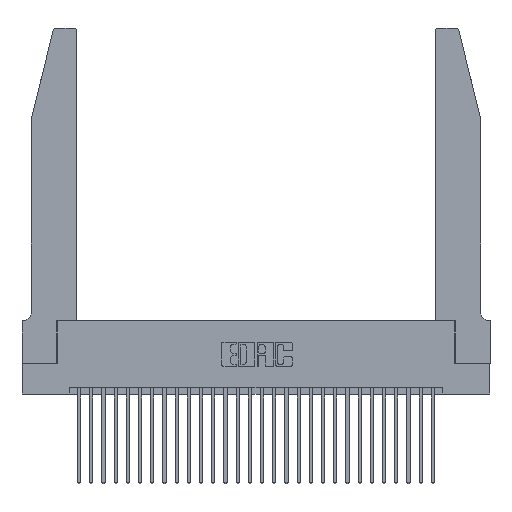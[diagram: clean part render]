
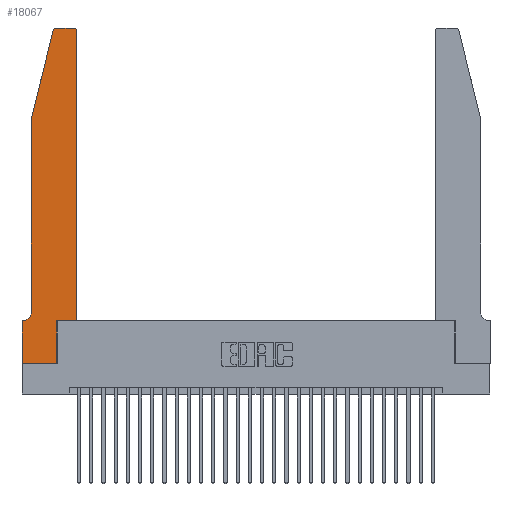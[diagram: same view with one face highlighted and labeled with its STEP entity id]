
A CAD part, top view. The second image highlights one B-rep face of the part: STEP entity #18067.
In plain terms, the highlighted planar face has unit normal (0, 0, 1).
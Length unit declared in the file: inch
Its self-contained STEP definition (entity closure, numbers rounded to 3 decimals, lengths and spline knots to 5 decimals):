
#1061 = VECTOR ( 'NONE', #6796, 39.37008 ) ;
#1632 = ORIENTED_EDGE ( 'NONE', *, *, #29588, .T. ) ;
#1982 = LINE ( 'NONE', #19739, #25883 ) ;
#2063 = CARTESIAN_POINT ( 'NONE',  ( 0.2605, 2.75, 0.37 ) ) ;
#2290 = ORIENTED_EDGE ( 'NONE', *, *, #21706, .T. ) ;
#3856 = CARTESIAN_POINT ( 'NONE',  ( 0.4205, 2.72, 0.37 ) ) ;
#4141 = DIRECTION ( 'NONE',  ( 0., -1., 0. ) ) ;
#5134 = VECTOR ( 'NONE', #19343, 39.37008 ) ;
#5338 = DIRECTION ( 'NONE',  ( 1., 0., 0. ) ) ;
#5572 = DIRECTION ( 'NONE',  ( -0.239, -0.971, 0. ) ) ;
#6156 = CARTESIAN_POINT ( 'NONE',  ( 0.4205, 2.75, 0.37 ) ) ;
#6493 = EDGE_CURVE ( 'NONE', #22655, #26320, #8952, .T. ) ;
#6659 = ORIENTED_EDGE ( 'NONE', *, *, #19389, .T. ) ;
#6733 = CARTESIAN_POINT ( 'NONE',  ( 0.284, 2.72, 0.37 ) ) ;
#6796 = DIRECTION ( 'NONE',  ( 0., 1., 0. ) ) ;
#7118 = AXIS2_PLACEMENT_3D ( 'NONE', #3856, #22224, #20282 ) ;
#7209 = LINE ( 'NONE', #25021, #1061 ) ;
#7869 = VERTEX_POINT ( 'NONE', #20244 ) ;
#8252 = CARTESIAN_POINT ( 'NONE',  ( 0.4505, 0.35, 0.37 ) ) ;
#8328 = AXIS2_PLACEMENT_3D ( 'NONE', #6733, #25265, #27579 ) ;
#8332 = DIRECTION ( 'NONE',  ( -1., 0., 0. ) ) ;
#8952 = LINE ( 'NONE', #11837, #28166 ) ;
#9017 = VERTEX_POINT ( 'NONE', #27501 ) ;
#9073 = VERTEX_POINT ( 'NONE', #13905 ) ;
#9078 = ORIENTED_EDGE ( 'NONE', *, *, #29546, .T. ) ;
#9203 = VECTOR ( 'NONE', #5338, 39.37008 ) ;
#9362 = VECTOR ( 'NONE', #11116, 39.37008 ) ;
#9477 = LINE ( 'NONE', #23958, #5134 ) ;
#9739 = EDGE_CURVE ( 'NONE', #13799, #22655, #9477, .T. ) ;
#9855 = CARTESIAN_POINT ( 'NONE',  ( 0., 0., 0.37 ) ) ;
#10223 = CARTESIAN_POINT ( 'NONE',  ( 0.25487, 2.72718, 0.37 ) ) ;
#10576 = ORIENTED_EDGE ( 'NONE', *, *, #16892, .T. ) ;
#11116 = DIRECTION ( 'NONE',  ( -1., 0., 0. ) ) ;
#11837 = CARTESIAN_POINT ( 'NONE',  ( 0.4505, 0.35, 0.37 ) ) ;
#12440 = CARTESIAN_POINT ( 'NONE',  ( 0.0755, 2., 0.37 ) ) ;
#12889 = CARTESIAN_POINT ( 'NONE',  ( 0.0055, 0.42, 0.37 ) ) ;
#13212 = VECTOR ( 'NONE', #4141, 39.37008 ) ;
#13799 = VERTEX_POINT ( 'NONE', #24764 ) ;
#13905 = CARTESIAN_POINT ( 'NONE',  ( 0., 0.35, 0.37 ) ) ;
#14113 = CIRCLE ( 'NONE', #8328, 0.03 ) ;
#14149 = EDGE_CURVE ( 'NONE', #21076, #9017, #16489, .T. ) ;
#14262 = CARTESIAN_POINT ( 'NONE',  ( 0.4505, 2.72, 0.37 ) ) ;
#14494 = VERTEX_POINT ( 'NONE', #6156 ) ;
#14792 = VECTOR ( 'NONE', #5572, 39.37008 ) ;
#15273 = ORIENTED_EDGE ( 'NONE', *, *, #6493, .T. ) ;
#15652 = CARTESIAN_POINT ( 'NONE',  ( 0., 0., 0.37 ) ) ;
#15943 = DIRECTION ( 'NONE',  ( 0., 0., 1. ) ) ;
#16089 = CIRCLE ( 'NONE', #7118, 0.03 ) ;
#16137 = ORIENTED_EDGE ( 'NONE', *, *, #25163, .T. ) ;
#16489 = CIRCLE ( 'NONE', #19311, 0.07 ) ;
#16553 = VERTEX_POINT ( 'NONE', #10223 ) ;
#16892 = EDGE_CURVE ( 'NONE', #16553, #23480, #28209, .T. ) ;
#17016 = ORIENTED_EDGE ( 'NONE', *, *, #29113, .T. ) ;
#17383 = DIRECTION ( 'NONE',  ( 0., 0., -1. ) ) ;
#17653 = PLANE ( 'NONE',  #24280 ) ;
#17777 = CARTESIAN_POINT ( 'NONE',  ( 0.0755, 0.42, 0.37 ) ) ;
#17938 = CARTESIAN_POINT ( 'NONE',  ( 0.0755, 2., 0.37 ) ) ;
#18067 = ADVANCED_FACE ( 'NONE', ( #21956 ), #17653, .T. ) ;
#19130 = CARTESIAN_POINT ( 'NONE',  ( 0.0755, 2., 0.37 ) ) ;
#19247 = ORIENTED_EDGE ( 'NONE', *, *, #14149, .T. ) ;
#19311 = AXIS2_PLACEMENT_3D ( 'NONE', #12889, #17383, #24340 ) ;
#19343 = DIRECTION ( 'NONE',  ( 1., 0., 0. ) ) ;
#19389 = EDGE_CURVE ( 'NONE', #23480, #21076, #27340, .T. ) ;
#19671 = DIRECTION ( 'NONE',  ( 0., 1., 0. ) ) ;
#19739 = CARTESIAN_POINT ( 'NONE',  ( 0.0755, 0.35, 0.37 ) ) ;
#20244 = CARTESIAN_POINT ( 'NONE',  ( 0., 0., 0.37 ) ) ;
#20282 = DIRECTION ( 'NONE',  ( 1., 0., 0. ) ) ;
#20505 = DIRECTION ( 'NONE',  ( 1., 0., 0. ) ) ;
#20700 = VECTOR ( 'NONE', #23064, 39.37008 ) ;
#21076 = VERTEX_POINT ( 'NONE', #17777 ) ;
#21661 = ORIENTED_EDGE ( 'NONE', *, *, #25024, .T. ) ;
#21706 = EDGE_CURVE ( 'NONE', #9073, #7869, #26887, .T. ) ;
#21956 = FACE_OUTER_BOUND ( 'NONE', #27781, .T. ) ;
#22224 = DIRECTION ( 'NONE',  ( 0., 0., 1. ) ) ;
#22655 = VERTEX_POINT ( 'NONE', #8252 ) ;
#23064 = DIRECTION ( 'NONE',  ( 0., -1., 0. ) ) ;
#23480 = VERTEX_POINT ( 'NONE', #19130 ) ;
#23958 = CARTESIAN_POINT ( 'NONE',  ( 0.4505, 0.35, 0.37 ) ) ;
#24066 = LINE ( 'NONE', #9855, #9203 ) ;
#24280 = AXIS2_PLACEMENT_3D ( 'NONE', #27836, #15943, #20505 ) ;
#24340 = DIRECTION ( 'NONE',  ( -1., 0., 0. ) ) ;
#24466 = EDGE_CURVE ( 'NONE', #26320, #14494, #16089, .T. ) ;
#24531 = VERTEX_POINT ( 'NONE', #24996 ) ;
#24764 = CARTESIAN_POINT ( 'NONE',  ( 0.2865, 0.35, 0.37 ) ) ;
#24996 = CARTESIAN_POINT ( 'NONE',  ( 0.2865, 0., 0.37 ) ) ;
#25021 = CARTESIAN_POINT ( 'NONE',  ( 0.2865, 0.35, 0.37 ) ) ;
#25024 = EDGE_CURVE ( 'NONE', #7869, #24531, #24066, .T. ) ;
#25163 = EDGE_CURVE ( 'NONE', #9017, #9073, #1982, .T. ) ;
#25265 = DIRECTION ( 'NONE',  ( 0., 0., 1. ) ) ;
#25883 = VECTOR ( 'NONE', #8332, 39.37008 ) ;
#26320 = VERTEX_POINT ( 'NONE', #14262 ) ;
#26405 = LINE ( 'NONE', #2063, #9362 ) ;
#26887 = LINE ( 'NONE', #15652, #20700 ) ;
#26948 = CARTESIAN_POINT ( 'NONE',  ( 0.284, 2.75, 0.37 ) ) ;
#27340 = LINE ( 'NONE', #17938, #13212 ) ;
#27501 = CARTESIAN_POINT ( 'NONE',  ( 0.0055, 0.35, 0.37 ) ) ;
#27579 = DIRECTION ( 'NONE',  ( 1., 0., 0. ) ) ;
#27781 = EDGE_LOOP ( 'NONE', ( #9078, #17016, #10576, #6659, #19247, #16137, #2290, #21661, #1632, #29381, #15273, #29273 ) ) ;
#27836 = CARTESIAN_POINT ( 'NONE',  ( 0., 0.35, 0.37 ) ) ;
#28166 = VECTOR ( 'NONE', #19671, 39.37008 ) ;
#28209 = LINE ( 'NONE', #12440, #14792 ) ;
#28903 = VERTEX_POINT ( 'NONE', #26948 ) ;
#29113 = EDGE_CURVE ( 'NONE', #28903, #16553, #14113, .T. ) ;
#29273 = ORIENTED_EDGE ( 'NONE', *, *, #24466, .T. ) ;
#29381 = ORIENTED_EDGE ( 'NONE', *, *, #9739, .T. ) ;
#29546 = EDGE_CURVE ( 'NONE', #14494, #28903, #26405, .T. ) ;
#29588 = EDGE_CURVE ( 'NONE', #24531, #13799, #7209, .T. ) ;
